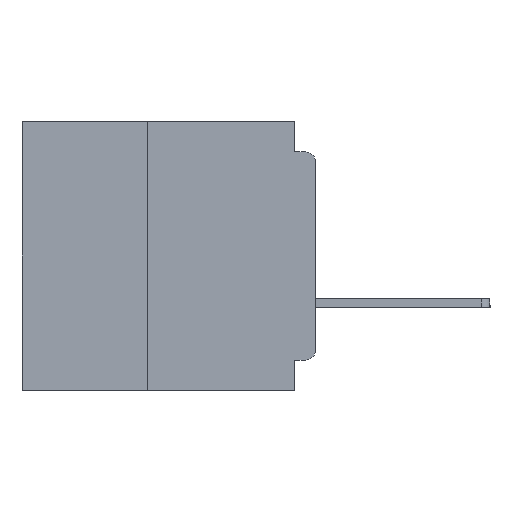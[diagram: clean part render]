
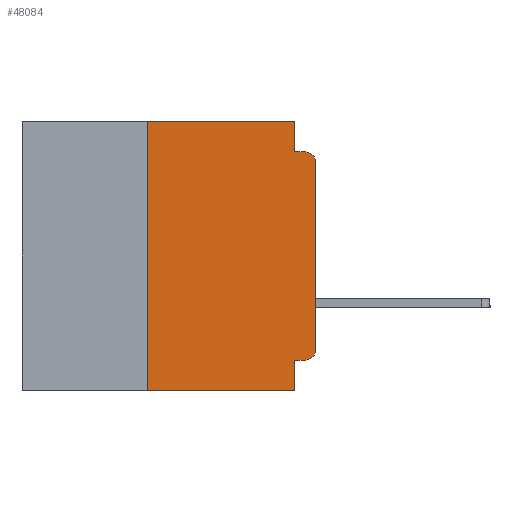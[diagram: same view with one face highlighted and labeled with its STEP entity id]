
A CAD part, left-side view. The second image highlights one B-rep face of the part: STEP entity #48084.
In plain terms, the highlighted planar face has unit normal (-1, 0, 0).
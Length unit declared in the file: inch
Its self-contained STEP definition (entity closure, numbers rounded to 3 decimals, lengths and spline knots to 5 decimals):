
#178 = LINE ( 'NONE', #36673, #41365 ) ;
#210 = ORIENTED_EDGE ( 'NONE', *, *, #9411, .T. ) ;
#216 = LINE ( 'NONE', #50800, #41394 ) ;
#453 = DIRECTION ( 'NONE',  ( 0., 0., -1. ) ) ;
#1919 = EDGE_CURVE ( 'NONE', #34794, #50833, #216, .T. ) ;
#3984 = DIRECTION ( 'NONE',  ( -1., 0., 0. ) ) ;
#4236 = VERTEX_POINT ( 'NONE', #42191 ) ;
#4531 = EDGE_CURVE ( 'NONE', #23610, #38862, #14512, .T. ) ;
#4891 = CARTESIAN_POINT ( 'NONE',  ( 0., 0.015, -0.06 ) ) ;
#4938 = LINE ( 'NONE', #14981, #26245 ) ;
#5637 = ORIENTED_EDGE ( 'NONE', *, *, #22869, .T. ) ;
#5704 = FACE_OUTER_BOUND ( 'NONE', #23849, .T. ) ;
#6075 = CARTESIAN_POINT ( 'NONE',  ( 0., 0., -0.045 ) ) ;
#6431 = VERTEX_POINT ( 'NONE', #14497 ) ;
#7111 = EDGE_CURVE ( 'NONE', #8124, #28263, #4938, .T. ) ;
#7408 = CARTESIAN_POINT ( 'NONE',  ( 0., 0.015, -0.355 ) ) ;
#8124 = VERTEX_POINT ( 'NONE', #34438 ) ;
#8328 = EDGE_CURVE ( 'NONE', #50833, #35544, #8818, .T. ) ;
#8818 = LINE ( 'NONE', #6075, #30033 ) ;
#9207 = DIRECTION ( 'NONE',  ( 0., 0., -1. ) ) ;
#9411 = EDGE_CURVE ( 'NONE', #8124, #12791, #41771, .T. ) ;
#10379 = DIRECTION ( 'NONE',  ( 0., -1., 0. ) ) ;
#12791 = VERTEX_POINT ( 'NONE', #21305 ) ;
#13220 = CARTESIAN_POINT ( 'NONE',  ( 0., 0.437, 0. ) ) ;
#14132 = ORIENTED_EDGE ( 'NONE', *, *, #4531, .F. ) ;
#14497 = CARTESIAN_POINT ( 'NONE',  ( 0., 0., -0.06 ) ) ;
#14512 = LINE ( 'NONE', #35867, #53996 ) ;
#14981 = CARTESIAN_POINT ( 'NONE',  ( 0., 0.25, -0.4 ) ) ;
#15264 = CARTESIAN_POINT ( 'NONE',  ( 0., 0.437, 0. ) ) ;
#15384 = CARTESIAN_POINT ( 'NONE',  ( 0., 0.25, 0. ) ) ;
#16052 = AXIS2_PLACEMENT_3D ( 'NONE', #29450, #3984, #33671 ) ;
#16109 = LINE ( 'NONE', #17595, #17443 ) ;
#17324 = PLANE ( 'NONE',  #45043 ) ;
#17443 = VECTOR ( 'NONE', #47063, 39.37008 ) ;
#17595 = CARTESIAN_POINT ( 'NONE',  ( 0., 0., 0. ) ) ;
#17620 = ORIENTED_EDGE ( 'NONE', *, *, #27644, .F. ) ;
#19157 = CARTESIAN_POINT ( 'NONE',  ( 0., 0.437, -0.4 ) ) ;
#19194 = CARTESIAN_POINT ( 'NONE',  ( 0., 0.031, -0.355 ) ) ;
#19274 = DIRECTION ( 'NONE',  ( 0., 0., 1. ) ) ;
#19853 = ORIENTED_EDGE ( 'NONE', *, *, #22764, .T. ) ;
#20764 = CARTESIAN_POINT ( 'NONE',  ( 0., 0.015, -0.045 ) ) ;
#21305 = CARTESIAN_POINT ( 'NONE',  ( 0., 0.031, -0.4 ) ) ;
#22764 = EDGE_CURVE ( 'NONE', #23610, #4236, #45139, .T. ) ;
#22869 = EDGE_CURVE ( 'NONE', #4236, #6431, #16109, .T. ) ;
#23610 = VERTEX_POINT ( 'NONE', #7408 ) ;
#23849 = EDGE_LOOP ( 'NONE', ( #5637, #52912, #36513, #44861, #17620, #41047, #210, #49662, #14132, #19853 ) ) ;
#26030 = DIRECTION ( 'NONE',  ( 1., 0., 0. ) ) ;
#26245 = VECTOR ( 'NONE', #19274, 39.37008 ) ;
#27644 = EDGE_CURVE ( 'NONE', #28263, #34794, #45304, .T. ) ;
#27699 = EDGE_CURVE ( 'NONE', #38862, #12791, #178, .T. ) ;
#28195 = CARTESIAN_POINT ( 'NONE',  ( 0., 0.031, 0. ) ) ;
#28263 = VERTEX_POINT ( 'NONE', #15384 ) ;
#29450 = CARTESIAN_POINT ( 'NONE',  ( 0., 0.015, -0.34 ) ) ;
#30033 = VECTOR ( 'NONE', #10379, 39.37008 ) ;
#30558 = VECTOR ( 'NONE', #44353, 39.37008 ) ;
#30765 = AXIS2_PLACEMENT_3D ( 'NONE', #4891, #34547, #9207 ) ;
#33671 = DIRECTION ( 'NONE',  ( 0., 0., -1. ) ) ;
#34438 = CARTESIAN_POINT ( 'NONE',  ( 0., 0.25, -0.4 ) ) ;
#34547 = DIRECTION ( 'NONE',  ( -1., 0., 0. ) ) ;
#34794 = VERTEX_POINT ( 'NONE', #28195 ) ;
#35544 = VERTEX_POINT ( 'NONE', #20764 ) ;
#35867 = CARTESIAN_POINT ( 'NONE',  ( 0., 0., -0.355 ) ) ;
#36310 = DIRECTION ( 'NONE',  ( 0., -1., 0. ) ) ;
#36513 = ORIENTED_EDGE ( 'NONE', *, *, #8328, .F. ) ;
#36673 = CARTESIAN_POINT ( 'NONE',  ( 0., 0.031, -0.4 ) ) ;
#38017 = EDGE_CURVE ( 'NONE', #6431, #35544, #49650, .T. ) ;
#38855 = CARTESIAN_POINT ( 'NONE',  ( 0., 0.031, -0.045 ) ) ;
#38862 = VERTEX_POINT ( 'NONE', #19194 ) ;
#40090 = DIRECTION ( 'NONE',  ( 0., 1., 0. ) ) ;
#41047 = ORIENTED_EDGE ( 'NONE', *, *, #7111, .F. ) ;
#41365 = VECTOR ( 'NONE', #53356, 39.37008 ) ;
#41394 = VECTOR ( 'NONE', #42401, 39.37008 ) ;
#41771 = LINE ( 'NONE', #19157, #30558 ) ;
#42191 = CARTESIAN_POINT ( 'NONE',  ( 0., 0., -0.34 ) ) ;
#42401 = DIRECTION ( 'NONE',  ( 0., 0., -1. ) ) ;
#43983 = VECTOR ( 'NONE', #36310, 39.37008 ) ;
#44353 = DIRECTION ( 'NONE',  ( 0., -1., 0. ) ) ;
#44861 = ORIENTED_EDGE ( 'NONE', *, *, #1919, .F. ) ;
#45043 = AXIS2_PLACEMENT_3D ( 'NONE', #13220, #26030, #453 ) ;
#45139 = CIRCLE ( 'NONE', #16052, 0.015 ) ;
#45304 = LINE ( 'NONE', #15264, #43983 ) ;
#47063 = DIRECTION ( 'NONE',  ( 0., 0., 1. ) ) ;
#48084 = ADVANCED_FACE ( 'NONE', ( #5704 ), #17324, .F. ) ;
#49650 = CIRCLE ( 'NONE', #30765, 0.015 ) ;
#49662 = ORIENTED_EDGE ( 'NONE', *, *, #27699, .F. ) ;
#50800 = CARTESIAN_POINT ( 'NONE',  ( 0., 0.031, 0. ) ) ;
#50833 = VERTEX_POINT ( 'NONE', #38855 ) ;
#52912 = ORIENTED_EDGE ( 'NONE', *, *, #38017, .T. ) ;
#53356 = DIRECTION ( 'NONE',  ( 0., 0., -1. ) ) ;
#53996 = VECTOR ( 'NONE', #40090, 39.37008 ) ;
